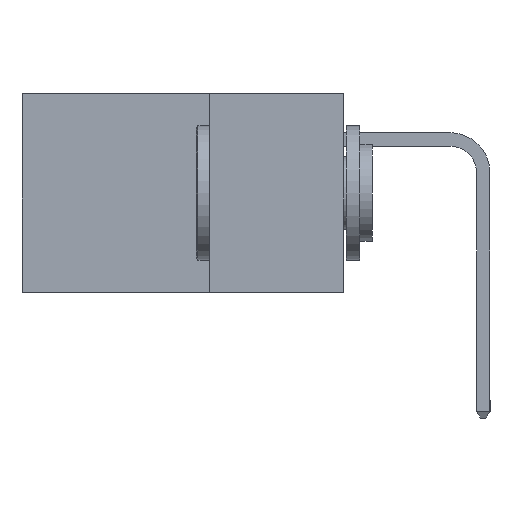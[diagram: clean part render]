
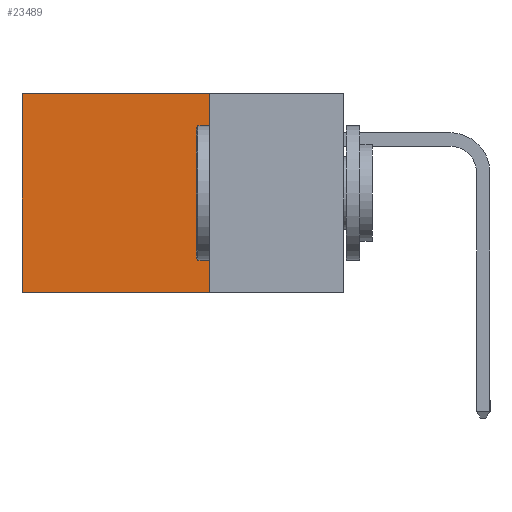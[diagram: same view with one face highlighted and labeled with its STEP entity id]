
A CAD part, left-side view. The second image highlights one B-rep face of the part: STEP entity #23489.
In plain terms, the highlighted planar face has unit normal (-1, 0, 0).
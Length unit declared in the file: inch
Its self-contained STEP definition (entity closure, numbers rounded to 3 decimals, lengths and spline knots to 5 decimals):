
#502 = CARTESIAN_POINT ( 'NONE',  ( 0.2615, 0.25, -0.37 ) ) ;
#670 = FACE_OUTER_BOUND ( 'NONE', #17514, .T. ) ;
#1975 = EDGE_CURVE ( 'NONE', #5953, #8038, #6856, .T. ) ;
#4518 = CARTESIAN_POINT ( 'NONE',  ( 0.2615, 0.25, -0.37 ) ) ;
#4598 = DIRECTION ( 'NONE',  ( 0., 0., -1. ) ) ;
#5023 = EDGE_CURVE ( 'NONE', #8038, #17050, #20379, .T. ) ;
#5059 = DIRECTION ( 'NONE',  ( 0., 1., 0. ) ) ;
#5435 = CARTESIAN_POINT ( 'NONE',  ( 0.2615, 0.6, 0. ) ) ;
#5953 = VERTEX_POINT ( 'NONE', #20008 ) ;
#6856 = LINE ( 'NONE', #9666, #11608 ) ;
#7286 = CARTESIAN_POINT ( 'NONE',  ( 0.2615, 0.6, -0.37 ) ) ;
#8038 = VERTEX_POINT ( 'NONE', #502 ) ;
#8262 = VECTOR ( 'NONE', #5059, 39.37008 ) ;
#8271 = ORIENTED_EDGE ( 'NONE', *, *, #5023, .F. ) ;
#9666 = CARTESIAN_POINT ( 'NONE',  ( 0.2615, 0.25, -0.37 ) ) ;
#10286 = VERTEX_POINT ( 'NONE', #5435 ) ;
#11608 = VECTOR ( 'NONE', #17830, 39.37008 ) ;
#11661 = EDGE_CURVE ( 'NONE', #5953, #10286, #19647, .T. ) ;
#12440 = ORIENTED_EDGE ( 'NONE', *, *, #1975, .F. ) ;
#12585 = PLANE ( 'NONE',  #17250 ) ;
#13626 = ORIENTED_EDGE ( 'NONE', *, *, #17535, .T. ) ;
#15394 = DIRECTION ( 'NONE',  ( 0., 0., -1. ) ) ;
#16637 = DIRECTION ( 'NONE',  ( 1., 0., 0. ) ) ;
#16741 = VECTOR ( 'NONE', #15394, 39.37008 ) ;
#17050 = VERTEX_POINT ( 'NONE', #17742 ) ;
#17250 = AXIS2_PLACEMENT_3D ( 'NONE', #4518, #16637, #4598 ) ;
#17514 = EDGE_LOOP ( 'NONE', ( #13626, #8271, #12440, #20183 ) ) ;
#17535 = EDGE_CURVE ( 'NONE', #10286, #17050, #22086, .T. ) ;
#17742 = CARTESIAN_POINT ( 'NONE',  ( 0.2615, 0.6, -0.37 ) ) ;
#17830 = DIRECTION ( 'NONE',  ( 0., 0., -1. ) ) ;
#19151 = CARTESIAN_POINT ( 'NONE',  ( 0.2615, 0.25, 0. ) ) ;
#19647 = LINE ( 'NONE', #19151, #8262 ) ;
#20008 = CARTESIAN_POINT ( 'NONE',  ( 0.2615, 0.25, 0. ) ) ;
#20183 = ORIENTED_EDGE ( 'NONE', *, *, #11661, .T. ) ;
#20379 = LINE ( 'NONE', #25189, #25038 ) ;
#21194 = DIRECTION ( 'NONE',  ( 0., 1., 0. ) ) ;
#22086 = LINE ( 'NONE', #7286, #16741 ) ;
#23489 = ADVANCED_FACE ( 'NONE', ( #670 ), #12585, .F. ) ;
#25038 = VECTOR ( 'NONE', #21194, 39.37008 ) ;
#25189 = CARTESIAN_POINT ( 'NONE',  ( 0.2615, 0.25, -0.37 ) ) ;
